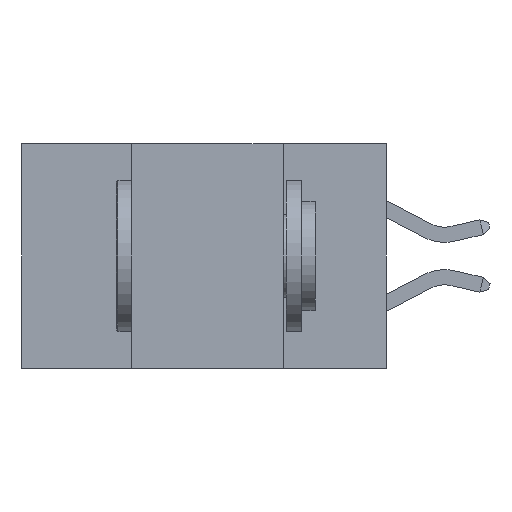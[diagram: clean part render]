
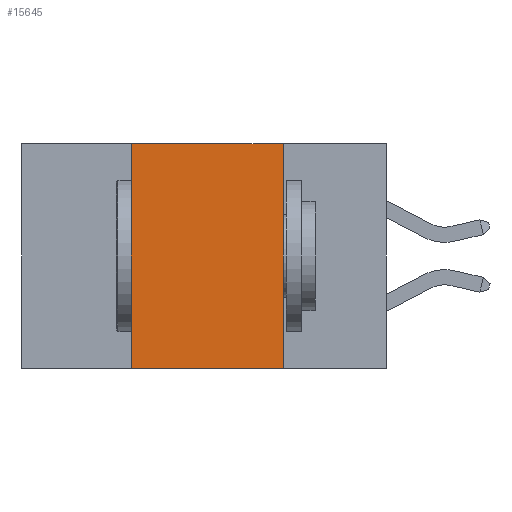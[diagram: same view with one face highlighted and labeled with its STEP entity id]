
A CAD part, left-side view. The second image highlights one B-rep face of the part: STEP entity #15645.
In plain terms, the highlighted planar face has unit normal (-1, 0, 0).
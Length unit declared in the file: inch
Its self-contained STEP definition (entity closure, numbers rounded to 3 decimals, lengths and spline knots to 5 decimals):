
#597 = FACE_OUTER_BOUND ( 'NONE', #2142, .T. ) ;
#684 = CARTESIAN_POINT ( 'NONE',  ( 0., 0.42, -0.37 ) ) ;
#879 = EDGE_CURVE ( 'NONE', #8943, #10699, #4311, .T. ) ;
#1139 = VECTOR ( 'NONE', #4480, 39.37008 ) ;
#1640 = LINE ( 'NONE', #7527, #15019 ) ;
#1908 = CARTESIAN_POINT ( 'NONE',  ( 0., 0.17, 0. ) ) ;
#2135 = CARTESIAN_POINT ( 'NONE',  ( 0., 0.6, 0. ) ) ;
#2142 = EDGE_LOOP ( 'NONE', ( #11207, #6816, #7237, #2848 ) ) ;
#2707 = VECTOR ( 'NONE', #6227, 39.37008 ) ;
#2848 = ORIENTED_EDGE ( 'NONE', *, *, #11903, .T. ) ;
#4311 = LINE ( 'NONE', #12764, #2707 ) ;
#4480 = DIRECTION ( 'NONE',  ( 0., -1., 0. ) ) ;
#5010 = VECTOR ( 'NONE', #16336, 39.37008 ) ;
#5308 = VERTEX_POINT ( 'NONE', #16145 ) ;
#6227 = DIRECTION ( 'NONE',  ( 0., 0., 1. ) ) ;
#6332 = CARTESIAN_POINT ( 'NONE',  ( 0., 0.17, 0. ) ) ;
#6816 = ORIENTED_EDGE ( 'NONE', *, *, #14607, .F. ) ;
#7237 = ORIENTED_EDGE ( 'NONE', *, *, #879, .F. ) ;
#7527 = CARTESIAN_POINT ( 'NONE',  ( 0., 0.6, 0. ) ) ;
#8433 = LINE ( 'NONE', #1908, #5010 ) ;
#8556 = DIRECTION ( 'NONE',  ( 0., 0., -1. ) ) ;
#8943 = VERTEX_POINT ( 'NONE', #684 ) ;
#9500 = CARTESIAN_POINT ( 'NONE',  ( 0., 0.6, -0.37 ) ) ;
#9789 = DIRECTION ( 'NONE',  ( 1., 0., 0. ) ) ;
#10699 = VERTEX_POINT ( 'NONE', #15546 ) ;
#11207 = ORIENTED_EDGE ( 'NONE', *, *, #16792, .F. ) ;
#11291 = DIRECTION ( 'NONE',  ( 0., -1., 0. ) ) ;
#11903 = EDGE_CURVE ( 'NONE', #8943, #5308, #12472, .T. ) ;
#12472 = LINE ( 'NONE', #9500, #1139 ) ;
#12764 = CARTESIAN_POINT ( 'NONE',  ( 0., 0.42, 0. ) ) ;
#13071 = VERTEX_POINT ( 'NONE', #6332 ) ;
#14607 = EDGE_CURVE ( 'NONE', #10699, #13071, #1640, .T. ) ;
#15019 = VECTOR ( 'NONE', #11291, 39.37008 ) ;
#15229 = AXIS2_PLACEMENT_3D ( 'NONE', #2135, #9789, #8556 ) ;
#15546 = CARTESIAN_POINT ( 'NONE',  ( 0., 0.42, 0. ) ) ;
#15645 = ADVANCED_FACE ( 'NONE', ( #597 ), #16388, .F. ) ;
#16145 = CARTESIAN_POINT ( 'NONE',  ( 0., 0.17, -0.37 ) ) ;
#16336 = DIRECTION ( 'NONE',  ( 0., 0., -1. ) ) ;
#16388 = PLANE ( 'NONE',  #15229 ) ;
#16792 = EDGE_CURVE ( 'NONE', #13071, #5308, #8433, .T. ) ;
